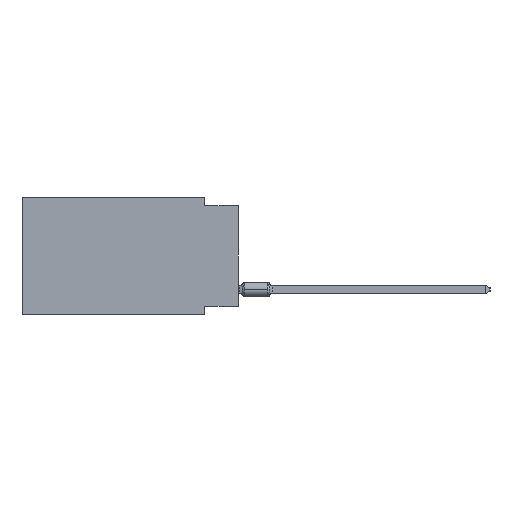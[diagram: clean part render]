
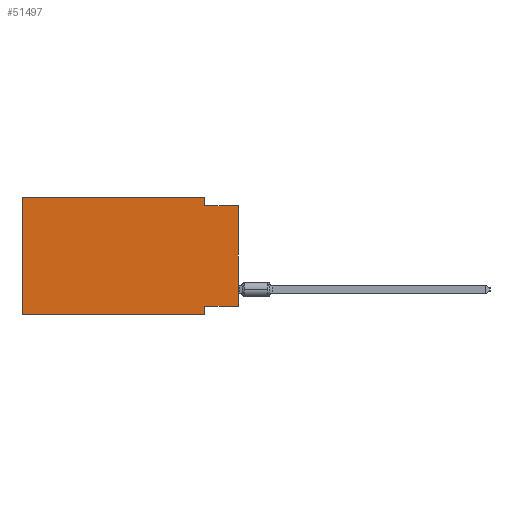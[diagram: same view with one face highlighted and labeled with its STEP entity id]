
A CAD part, left-side view. The second image highlights one B-rep face of the part: STEP entity #51497.
In plain terms, the highlighted planar face has unit normal (-1, 0, 0).
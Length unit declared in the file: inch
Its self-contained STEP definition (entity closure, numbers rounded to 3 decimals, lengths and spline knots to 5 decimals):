
#1052 = ORIENTED_EDGE ( 'NONE', *, *, #51236, .F. ) ;
#2428 = VECTOR ( 'NONE', #31097, 39.37008 ) ;
#4764 = CARTESIAN_POINT ( 'NONE',  ( 0., 0.645, 0. ) ) ;
#5206 = LINE ( 'NONE', #22239, #2428 ) ;
#6341 = EDGE_CURVE ( 'NONE', #57444, #113847, #5206, .T. ) ;
#8695 = EDGE_CURVE ( 'NONE', #40215, #84633, #115616, .T. ) ;
#9337 = VECTOR ( 'NONE', #16633, 39.37008 ) ;
#10796 = VERTEX_POINT ( 'NONE', #32157 ) ;
#12133 = LINE ( 'NONE', #100342, #21790 ) ;
#13748 = CARTESIAN_POINT ( 'NONE',  ( 0., 0.645, 0. ) ) ;
#14664 = CARTESIAN_POINT ( 'NONE',  ( 0., 0., -0.025 ) ) ;
#14685 = CARTESIAN_POINT ( 'NONE',  ( 0., 0.645, -0.35 ) ) ;
#14828 = CARTESIAN_POINT ( 'NONE',  ( 0., 0., 0. ) ) ;
#16228 = VECTOR ( 'NONE', #111315, 39.37008 ) ;
#16633 = DIRECTION ( 'NONE',  ( 0., 1., 0. ) ) ;
#17034 = LINE ( 'NONE', #25313, #100376 ) ;
#20104 = DIRECTION ( 'NONE',  ( 0., -1., 0. ) ) ;
#21790 = VECTOR ( 'NONE', #47413, 39.37008 ) ;
#22239 = CARTESIAN_POINT ( 'NONE',  ( 0., 0.645, 0. ) ) ;
#22281 = DIRECTION ( 'NONE',  ( 0., 0., -1. ) ) ;
#25313 = CARTESIAN_POINT ( 'NONE',  ( 0., 0.1, -0.35 ) ) ;
#26919 = EDGE_CURVE ( 'NONE', #113847, #61427, #51168, .T. ) ;
#30802 = VERTEX_POINT ( 'NONE', #96146 ) ;
#31097 = DIRECTION ( 'NONE',  ( 0., 0., 1. ) ) ;
#31810 = ORIENTED_EDGE ( 'NONE', *, *, #35401, .F. ) ;
#32157 = CARTESIAN_POINT ( 'NONE',  ( 0., 0.1, -0.35 ) ) ;
#35061 = EDGE_CURVE ( 'NONE', #57444, #10796, #12133, .T. ) ;
#35401 = EDGE_CURVE ( 'NONE', #61427, #40215, #60073, .T. ) ;
#40215 = VERTEX_POINT ( 'NONE', #47189 ) ;
#43040 = CARTESIAN_POINT ( 'NONE',  ( 0., 0.1, 0. ) ) ;
#45238 = DIRECTION ( 'NONE',  ( 0., 0., -1. ) ) ;
#46242 = EDGE_CURVE ( 'NONE', #51697, #84633, #95412, .T. ) ;
#47189 = CARTESIAN_POINT ( 'NONE',  ( 0., 0.1, -0.025 ) ) ;
#47413 = DIRECTION ( 'NONE',  ( 0., -1., 0. ) ) ;
#47534 = ORIENTED_EDGE ( 'NONE', *, *, #8695, .F. ) ;
#51168 = LINE ( 'NONE', #4764, #56570 ) ;
#51236 = EDGE_CURVE ( 'NONE', #51697, #30802, #53090, .T. ) ;
#51497 = ADVANCED_FACE ( 'NONE', ( #84635 ), #67006, .F. ) ;
#51697 = VERTEX_POINT ( 'NONE', #96951 ) ;
#52817 = ORIENTED_EDGE ( 'NONE', *, *, #6341, .F. ) ;
#53090 = LINE ( 'NONE', #98960, #9337 ) ;
#54415 = AXIS2_PLACEMENT_3D ( 'NONE', #102876, #99512, #22281 ) ;
#56570 = VECTOR ( 'NONE', #87040, 39.37008 ) ;
#57444 = VERTEX_POINT ( 'NONE', #14685 ) ;
#60073 = LINE ( 'NONE', #104801, #16228 ) ;
#61427 = VERTEX_POINT ( 'NONE', #43040 ) ;
#67006 = PLANE ( 'NONE',  #54415 ) ;
#68063 = ORIENTED_EDGE ( 'NONE', *, *, #46242, .T. ) ;
#68950 = DIRECTION ( 'NONE',  ( 0., 0., 1. ) ) ;
#69458 = EDGE_LOOP ( 'NONE', ( #68063, #47534, #31810, #81984, #52817, #89180, #101773, #1052 ) ) ;
#81984 = ORIENTED_EDGE ( 'NONE', *, *, #26919, .F. ) ;
#84633 = VERTEX_POINT ( 'NONE', #14664 ) ;
#84635 = FACE_OUTER_BOUND ( 'NONE', #69458, .T. ) ;
#85805 = VECTOR ( 'NONE', #68950, 39.37008 ) ;
#87040 = DIRECTION ( 'NONE',  ( 0., -1., 0. ) ) ;
#89180 = ORIENTED_EDGE ( 'NONE', *, *, #35061, .T. ) ;
#93783 = VECTOR ( 'NONE', #20104, 39.37008 ) ;
#95412 = LINE ( 'NONE', #14828, #85805 ) ;
#96146 = CARTESIAN_POINT ( 'NONE',  ( 0., 0.1, -0.325 ) ) ;
#96814 = CARTESIAN_POINT ( 'NONE',  ( 0., 0., -0.025 ) ) ;
#96951 = CARTESIAN_POINT ( 'NONE',  ( 0., 0., -0.325 ) ) ;
#98960 = CARTESIAN_POINT ( 'NONE',  ( 0., 0., -0.325 ) ) ;
#99512 = DIRECTION ( 'NONE',  ( 1., 0., 0. ) ) ;
#100342 = CARTESIAN_POINT ( 'NONE',  ( 0., 0.645, -0.35 ) ) ;
#100376 = VECTOR ( 'NONE', #45238, 39.37008 ) ;
#101773 = ORIENTED_EDGE ( 'NONE', *, *, #111890, .F. ) ;
#102876 = CARTESIAN_POINT ( 'NONE',  ( 0., 0.645, 0. ) ) ;
#104801 = CARTESIAN_POINT ( 'NONE',  ( 0., 0.1, 0. ) ) ;
#111315 = DIRECTION ( 'NONE',  ( 0., 0., -1. ) ) ;
#111890 = EDGE_CURVE ( 'NONE', #30802, #10796, #17034, .T. ) ;
#113847 = VERTEX_POINT ( 'NONE', #13748 ) ;
#115616 = LINE ( 'NONE', #96814, #93783 ) ;
